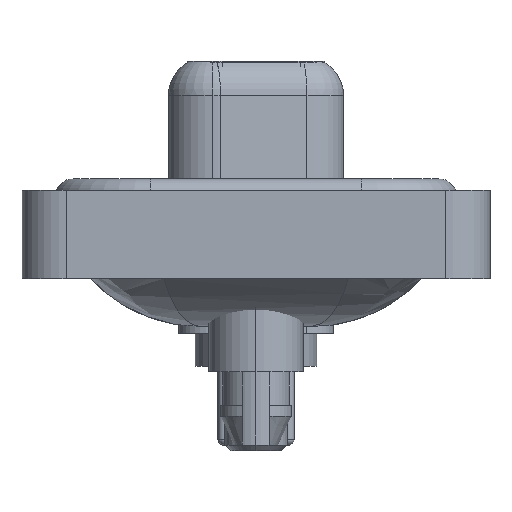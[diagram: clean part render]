
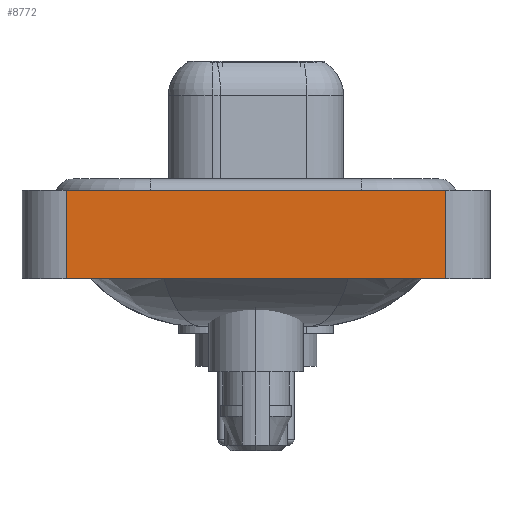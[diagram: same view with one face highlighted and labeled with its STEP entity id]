
A CAD part, left-side view. The second image highlights one B-rep face of the part: STEP entity #8772.
In plain terms, the highlighted planar face has unit normal (-1, 0, 0).
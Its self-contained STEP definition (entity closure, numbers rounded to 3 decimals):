
#127 = CARTESIAN_POINT ( 'NONE',  ( -7.35, -8.55, 0.4 ) ) ;
#502 = VECTOR ( 'NONE', #5205, 1000. ) ;
#1307 = VERTEX_POINT ( 'NONE', #127 ) ;
#1574 = LINE ( 'NONE', #8251, #21088 ) ;
#1627 = EDGE_CURVE ( 'NONE', #17443, #1307, #5096, .T. ) ;
#2235 = EDGE_LOOP ( 'NONE', ( #2841, #19909, #9962, #3953 ) ) ;
#2841 = ORIENTED_EDGE ( 'NONE', *, *, #21250, .T. ) ;
#3953 = ORIENTED_EDGE ( 'NONE', *, *, #10443, .T. ) ;
#4221 = DIRECTION ( 'NONE',  ( 0., 0., 1. ) ) ;
#5096 = LINE ( 'NONE', #16599, #502 ) ;
#5205 = DIRECTION ( 'NONE',  ( 0., -1., 0. ) ) ;
#6950 = FACE_OUTER_BOUND ( 'NONE', #2235, .T. ) ;
#7039 = LINE ( 'NONE', #20071, #13677 ) ;
#8026 = AXIS2_PLACEMENT_3D ( 'NONE', #18550, #16690, #17127 ) ;
#8251 = CARTESIAN_POINT ( 'NONE',  ( -7.35, 8.55, -3.6 ) ) ;
#8480 = PLANE ( 'NONE',  #8026 ) ;
#8772 = ADVANCED_FACE ( 'NONE', ( #6950 ), #8480, .T. ) ;
#9962 = ORIENTED_EDGE ( 'NONE', *, *, #13265, .F. ) ;
#10443 = EDGE_CURVE ( 'NONE', #11079, #16207, #7039, .T. ) ;
#10497 = CARTESIAN_POINT ( 'NONE',  ( -7.35, -8.55, -3.6 ) ) ;
#11079 = VERTEX_POINT ( 'NONE', #15957 ) ;
#11152 = CARTESIAN_POINT ( 'NONE',  ( -7.35, 8.55, 0.4 ) ) ;
#11730 = DIRECTION ( 'NONE',  ( 0., -1., 0. ) ) ;
#13265 = EDGE_CURVE ( 'NONE', #11079, #17443, #1574, .T. ) ;
#13677 = VECTOR ( 'NONE', #11730, 1000. ) ;
#14179 = CARTESIAN_POINT ( 'NONE',  ( -7.35, -8.55, -3.6 ) ) ;
#14931 = DIRECTION ( 'NONE',  ( 0., 0., 1. ) ) ;
#15941 = LINE ( 'NONE', #14179, #17757 ) ;
#15957 = CARTESIAN_POINT ( 'NONE',  ( -7.35, 8.55, -3.6 ) ) ;
#16207 = VERTEX_POINT ( 'NONE', #10497 ) ;
#16599 = CARTESIAN_POINT ( 'NONE',  ( -7.35, -8.55, 0.4 ) ) ;
#16690 = DIRECTION ( 'NONE',  ( -1., 0., 0. ) ) ;
#17127 = DIRECTION ( 'NONE',  ( 0., 0., 1. ) ) ;
#17443 = VERTEX_POINT ( 'NONE', #11152 ) ;
#17757 = VECTOR ( 'NONE', #4221, 1000. ) ;
#18550 = CARTESIAN_POINT ( 'NONE',  ( -7.35, -8.55, -3.6 ) ) ;
#19909 = ORIENTED_EDGE ( 'NONE', *, *, #1627, .F. ) ;
#20071 = CARTESIAN_POINT ( 'NONE',  ( -7.35, -8.55, -3.6 ) ) ;
#21088 = VECTOR ( 'NONE', #14931, 1000. ) ;
#21250 = EDGE_CURVE ( 'NONE', #16207, #1307, #15941, .T. ) ;
